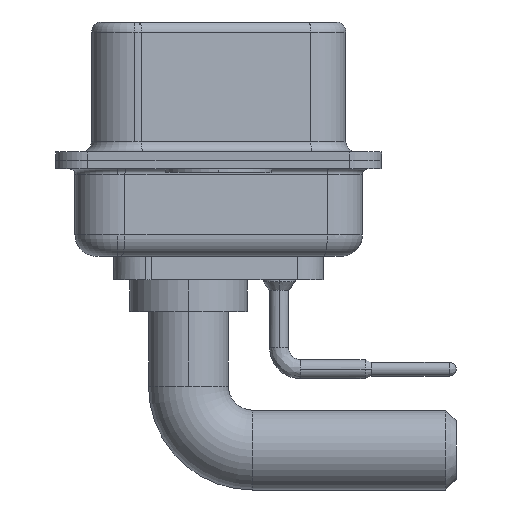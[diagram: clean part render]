
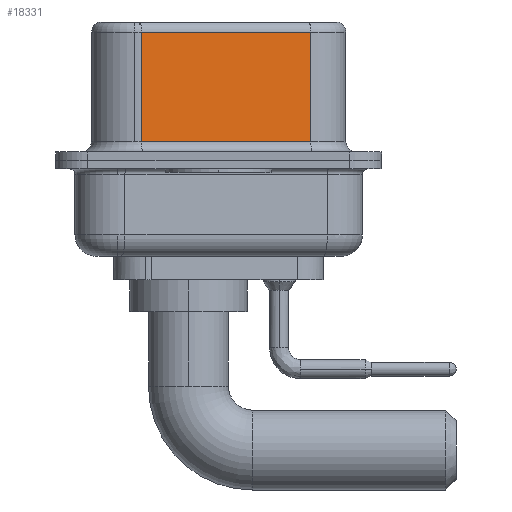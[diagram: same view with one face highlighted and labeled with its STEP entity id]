
A CAD part, left-side view. The second image highlights one B-rep face of the part: STEP entity #18331.
In plain terms, the highlighted planar face has unit normal (-0.985, -0.174, 0).
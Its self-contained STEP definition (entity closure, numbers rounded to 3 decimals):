
#557 = FACE_OUTER_BOUND ( 'NONE', #18611, .T. ) ;
#704 = EDGE_CURVE ( 'NONE', #20018, #4774, #16739, .T. ) ;
#1076 = CARTESIAN_POINT ( 'NONE',  ( 5.132, -4.322, 6.02 ) ) ;
#1375 = DIRECTION ( 'NONE',  ( 0.174, -0.985, 0. ) ) ;
#2365 = LINE ( 'NONE', #9178, #9550 ) ;
#2593 = LINE ( 'NONE', #17889, #20739 ) ;
#3059 = CARTESIAN_POINT ( 'NONE',  ( 5.132, -4.322, 0.9 ) ) ;
#4162 = VECTOR ( 'NONE', #16419, 1000. ) ;
#4774 = VERTEX_POINT ( 'NONE', #10367 ) ;
#4936 = LINE ( 'NONE', #3059, #7554 ) ;
#7554 = VECTOR ( 'NONE', #1375, 1000. ) ;
#7680 = EDGE_CURVE ( 'NONE', #4774, #20146, #4936, .T. ) ;
#9178 = CARTESIAN_POINT ( 'NONE',  ( 5.132, -4.322, 6.02 ) ) ;
#9550 = VECTOR ( 'NONE', #14547, 1000. ) ;
#10053 = ORIENTED_EDGE ( 'NONE', *, *, #21321, .T. ) ;
#10367 = CARTESIAN_POINT ( 'NONE',  ( 3.73, 3.628, 0.9 ) ) ;
#11407 = CARTESIAN_POINT ( 'NONE',  ( 5.132, -4.322, 0.9 ) ) ;
#11951 = VERTEX_POINT ( 'NONE', #1076 ) ;
#12628 = PLANE ( 'NONE',  #13027 ) ;
#12789 = EDGE_CURVE ( 'NONE', #11951, #20146, #2593, .T. ) ;
#13027 = AXIS2_PLACEMENT_3D ( 'NONE', #17635, #17852, #21095 ) ;
#13792 = ORIENTED_EDGE ( 'NONE', *, *, #7680, .T. ) ;
#14504 = CARTESIAN_POINT ( 'NONE',  ( 3.73, 3.628, 6.02 ) ) ;
#14547 = DIRECTION ( 'NONE',  ( -0.174, 0.985, 0. ) ) ;
#14704 = ORIENTED_EDGE ( 'NONE', *, *, #12789, .F. ) ;
#16419 = DIRECTION ( 'NONE',  ( 0., 0., -1. ) ) ;
#16739 = LINE ( 'NONE', #20088, #4162 ) ;
#17551 = DIRECTION ( 'NONE',  ( 0., 0., -1. ) ) ;
#17635 = CARTESIAN_POINT ( 'NONE',  ( 5.132, -4.322, 6.52 ) ) ;
#17852 = DIRECTION ( 'NONE',  ( 0.985, 0.174, 0. ) ) ;
#17889 = CARTESIAN_POINT ( 'NONE',  ( 5.132, -4.322, 6.52 ) ) ;
#18331 = ADVANCED_FACE ( 'NONE', ( #557 ), #12628, .F. ) ;
#18611 = EDGE_LOOP ( 'NONE', ( #14704, #10053, #22045, #13792 ) ) ;
#20018 = VERTEX_POINT ( 'NONE', #14504 ) ;
#20088 = CARTESIAN_POINT ( 'NONE',  ( 3.73, 3.628, 6.52 ) ) ;
#20146 = VERTEX_POINT ( 'NONE', #11407 ) ;
#20739 = VECTOR ( 'NONE', #17551, 1000. ) ;
#21095 = DIRECTION ( 'NONE',  ( -0.174, 0.985, 0. ) ) ;
#21321 = EDGE_CURVE ( 'NONE', #11951, #20018, #2365, .T. ) ;
#22045 = ORIENTED_EDGE ( 'NONE', *, *, #704, .T. ) ;
